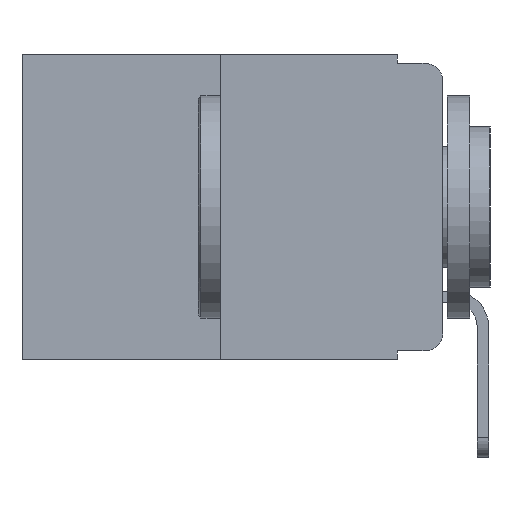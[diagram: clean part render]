
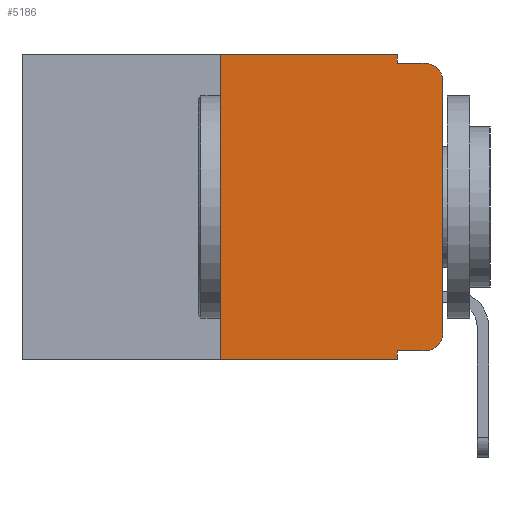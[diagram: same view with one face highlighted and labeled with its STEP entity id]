
A CAD part, left-side view. The second image highlights one B-rep face of the part: STEP entity #5186.
In plain terms, the highlighted planar face has unit normal (-1, 0, 0).
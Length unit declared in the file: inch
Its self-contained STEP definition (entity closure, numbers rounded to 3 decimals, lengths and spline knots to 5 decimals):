
#187 = DIRECTION ( 'NONE',  ( 0., -1., 0. ) ) ;
#430 = CARTESIAN_POINT ( 'NONE',  ( 0., 0., -0.313 ) ) ;
#438 = EDGE_CURVE ( 'NONE', #10024, #4728, #18789, .T. ) ;
#836 = VERTEX_POINT ( 'NONE', #4757 ) ;
#1121 = ORIENTED_EDGE ( 'NONE', *, *, #14072, .F. ) ;
#1242 = DIRECTION ( 'NONE',  ( 0., 0., 1. ) ) ;
#1403 = LINE ( 'NONE', #5612, #7299 ) ;
#1447 = VECTOR ( 'NONE', #1242, 39.37008 ) ;
#1558 = DIRECTION ( 'NONE',  ( 0., 0., -1. ) ) ;
#2178 = VECTOR ( 'NONE', #187, 39.37008 ) ;
#2319 = CARTESIAN_POINT ( 'NONE',  ( 0., 0.25, 0. ) ) ;
#2392 = ORIENTED_EDGE ( 'NONE', *, *, #11681, .T. ) ;
#2396 = CARTESIAN_POINT ( 'NONE',  ( 0., 0.051, -0.333 ) ) ;
#2680 = DIRECTION ( 'NONE',  ( 0., -1., 0. ) ) ;
#2965 = VERTEX_POINT ( 'NONE', #430 ) ;
#3258 = EDGE_CURVE ( 'NONE', #836, #13081, #11707, .T. ) ;
#3261 = VECTOR ( 'NONE', #18736, 39.37008 ) ;
#3314 = VERTEX_POINT ( 'NONE', #17691 ) ;
#3786 = ORIENTED_EDGE ( 'NONE', *, *, #9518, .F. ) ;
#4177 = ORIENTED_EDGE ( 'NONE', *, *, #438, .T. ) ;
#4454 = CARTESIAN_POINT ( 'NONE',  ( 0., 0.02, -0.313 ) ) ;
#4728 = VERTEX_POINT ( 'NONE', #5216 ) ;
#4757 = CARTESIAN_POINT ( 'NONE',  ( 0., 0.25, -0.343 ) ) ;
#5186 = ADVANCED_FACE ( 'NONE', ( #13640 ), #15595, .F. ) ;
#5216 = CARTESIAN_POINT ( 'NONE',  ( 0., 0.02, -0.333 ) ) ;
#5307 = CARTESIAN_POINT ( 'NONE',  ( 0., 0.02, -0.01 ) ) ;
#5528 = VECTOR ( 'NONE', #5587, 39.37008 ) ;
#5587 = DIRECTION ( 'NONE',  ( 0., 0., 1. ) ) ;
#5612 = CARTESIAN_POINT ( 'NONE',  ( 0., 0.473, -0.343 ) ) ;
#5639 = VECTOR ( 'NONE', #18338, 39.37008 ) ;
#6593 = DIRECTION ( 'NONE',  ( 0., 0., -1. ) ) ;
#6792 = VERTEX_POINT ( 'NONE', #14343 ) ;
#7037 = CARTESIAN_POINT ( 'NONE',  ( 0., 0.02, -0.03 ) ) ;
#7268 = DIRECTION ( 'NONE',  ( -1., 0., 0. ) ) ;
#7299 = VECTOR ( 'NONE', #2680, 39.37008 ) ;
#7628 = CARTESIAN_POINT ( 'NONE',  ( 0., 0.473, 0. ) ) ;
#8037 = ORIENTED_EDGE ( 'NONE', *, *, #11477, .F. ) ;
#8335 = CARTESIAN_POINT ( 'NONE',  ( 0., 0.25, 0. ) ) ;
#8618 = CARTESIAN_POINT ( 'NONE',  ( 0., 0.051, 0. ) ) ;
#8928 = VECTOR ( 'NONE', #10977, 39.37008 ) ;
#9153 = LINE ( 'NONE', #10786, #8928 ) ;
#9287 = CARTESIAN_POINT ( 'NONE',  ( 0., 0.051, -0.01 ) ) ;
#9484 = VERTEX_POINT ( 'NONE', #5307 ) ;
#9493 = EDGE_CURVE ( 'NONE', #4728, #2965, #13957, .T. ) ;
#9518 = EDGE_CURVE ( 'NONE', #3314, #9944, #18471, .T. ) ;
#9710 = AXIS2_PLACEMENT_3D ( 'NONE', #17115, #17051, #12721 ) ;
#9769 = EDGE_CURVE ( 'NONE', #2965, #6792, #11465, .T. ) ;
#9820 = VECTOR ( 'NONE', #16252, 39.37008 ) ;
#9944 = VERTEX_POINT ( 'NONE', #13877 ) ;
#10024 = VERTEX_POINT ( 'NONE', #2396 ) ;
#10786 = CARTESIAN_POINT ( 'NONE',  ( 0., 0.051, 0. ) ) ;
#10923 = ORIENTED_EDGE ( 'NONE', *, *, #15776, .F. ) ;
#10977 = DIRECTION ( 'NONE',  ( 0., 0., -1. ) ) ;
#11464 = AXIS2_PLACEMENT_3D ( 'NONE', #4454, #7268, #1558 ) ;
#11465 = LINE ( 'NONE', #14384, #1447 ) ;
#11477 = EDGE_CURVE ( 'NONE', #10024, #17424, #9153, .T. ) ;
#11528 = CARTESIAN_POINT ( 'NONE',  ( 0., 0.051, -0.343 ) ) ;
#11681 = EDGE_CURVE ( 'NONE', #836, #17424, #1403, .T. ) ;
#11707 = LINE ( 'NONE', #8335, #5528 ) ;
#12549 = CARTESIAN_POINT ( 'NONE',  ( 0., 0.051, -0.333 ) ) ;
#12721 = DIRECTION ( 'NONE',  ( 0., 0., -1. ) ) ;
#13081 = VERTEX_POINT ( 'NONE', #2319 ) ;
#13640 = FACE_OUTER_BOUND ( 'NONE', #17980, .T. ) ;
#13877 = CARTESIAN_POINT ( 'NONE',  ( 0., 0.051, -0.01 ) ) ;
#13957 = CIRCLE ( 'NONE', #11464, 0.02 ) ;
#14072 = EDGE_CURVE ( 'NONE', #9944, #9484, #16903, .T. ) ;
#14281 = DIRECTION ( 'NONE',  ( -1., 0., 0. ) ) ;
#14343 = CARTESIAN_POINT ( 'NONE',  ( 0., 0., -0.03 ) ) ;
#14384 = CARTESIAN_POINT ( 'NONE',  ( 0., 0., 0. ) ) ;
#14900 = ORIENTED_EDGE ( 'NONE', *, *, #3258, .F. ) ;
#15595 = PLANE ( 'NONE',  #9710 ) ;
#15776 = EDGE_CURVE ( 'NONE', #13081, #3314, #17050, .T. ) ;
#15907 = AXIS2_PLACEMENT_3D ( 'NONE', #7037, #14281, #6593 ) ;
#16252 = DIRECTION ( 'NONE',  ( 0., -1., 0. ) ) ;
#16742 = CIRCLE ( 'NONE', #15907, 0.02 ) ;
#16863 = ORIENTED_EDGE ( 'NONE', *, *, #17768, .T. ) ;
#16903 = LINE ( 'NONE', #9287, #2178 ) ;
#17050 = LINE ( 'NONE', #7628, #9820 ) ;
#17051 = DIRECTION ( 'NONE',  ( 1., 0., 0. ) ) ;
#17115 = CARTESIAN_POINT ( 'NONE',  ( 0., 0.473, 0. ) ) ;
#17424 = VERTEX_POINT ( 'NONE', #11528 ) ;
#17691 = CARTESIAN_POINT ( 'NONE',  ( 0., 0.051, 0. ) ) ;
#17768 = EDGE_CURVE ( 'NONE', #6792, #9484, #16742, .T. ) ;
#17980 = EDGE_LOOP ( 'NONE', ( #18127, #16863, #1121, #3786, #10923, #14900, #2392, #8037, #4177, #18399 ) ) ;
#18127 = ORIENTED_EDGE ( 'NONE', *, *, #9769, .T. ) ;
#18338 = DIRECTION ( 'NONE',  ( 0., -1., 0. ) ) ;
#18399 = ORIENTED_EDGE ( 'NONE', *, *, #9493, .T. ) ;
#18471 = LINE ( 'NONE', #8618, #3261 ) ;
#18736 = DIRECTION ( 'NONE',  ( 0., 0., -1. ) ) ;
#18789 = LINE ( 'NONE', #12549, #5639 ) ;
